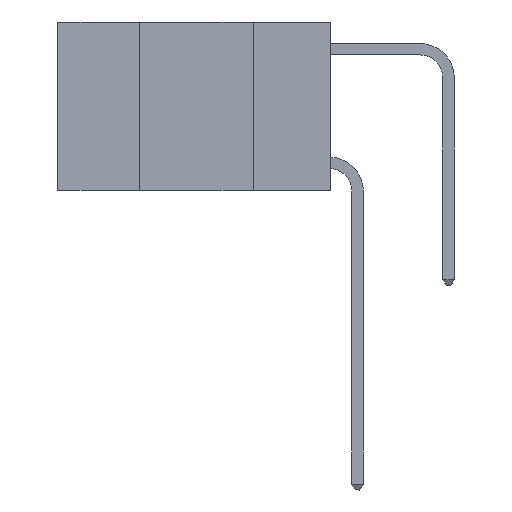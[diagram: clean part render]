
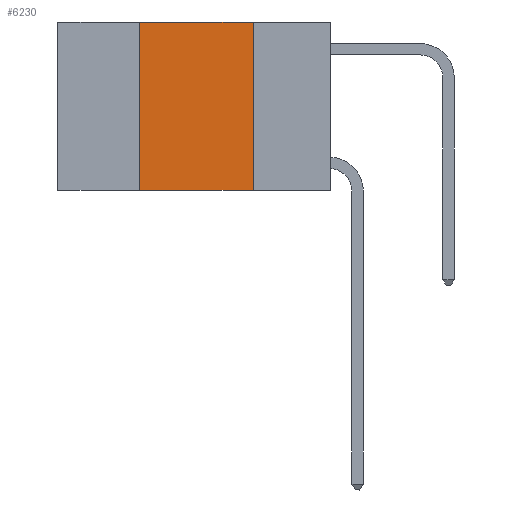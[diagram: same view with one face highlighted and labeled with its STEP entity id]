
A CAD part, left-side view. The second image highlights one B-rep face of the part: STEP entity #6230.
In plain terms, the highlighted planar face has unit normal (-1, 0, 0).
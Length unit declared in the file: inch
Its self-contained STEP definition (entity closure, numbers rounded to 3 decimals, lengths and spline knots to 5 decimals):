
#684 = CARTESIAN_POINT ( 'NONE',  ( 0., 0.6, 0. ) ) ;
#735 = CARTESIAN_POINT ( 'NONE',  ( 0., 0.42, -0.37 ) ) ;
#1099 = CARTESIAN_POINT ( 'NONE',  ( 0., 0.42, 0. ) ) ;
#1864 = EDGE_CURVE ( 'NONE', #15162, #2435, #2311, .T. ) ;
#2311 = LINE ( 'NONE', #20607, #16480 ) ;
#2326 = EDGE_CURVE ( 'NONE', #14271, #21335, #17048, .T. ) ;
#2435 = VERTEX_POINT ( 'NONE', #18611 ) ;
#2950 = VECTOR ( 'NONE', #8205, 39.37008 ) ;
#4415 = DIRECTION ( 'NONE',  ( 0., 0., -1. ) ) ;
#5647 = VECTOR ( 'NONE', #9096, 39.37008 ) ;
#5906 = EDGE_LOOP ( 'NONE', ( #21731, #22476, #23707, #12818 ) ) ;
#5960 = EDGE_CURVE ( 'NONE', #14271, #2435, #19722, .T. ) ;
#6230 = ADVANCED_FACE ( 'NONE', ( #9090 ), #20856, .F. ) ;
#6688 = VECTOR ( 'NONE', #23633, 39.37008 ) ;
#8205 = DIRECTION ( 'NONE',  ( 0., -1., 0. ) ) ;
#8472 = LINE ( 'NONE', #684, #2950 ) ;
#9090 = FACE_OUTER_BOUND ( 'NONE', #5906, .T. ) ;
#9096 = DIRECTION ( 'NONE',  ( 0., -1., 0. ) ) ;
#12818 = ORIENTED_EDGE ( 'NONE', *, *, #5960, .T. ) ;
#13279 = CARTESIAN_POINT ( 'NONE',  ( 0., 0.17, 0. ) ) ;
#14271 = VERTEX_POINT ( 'NONE', #735 ) ;
#15162 = VERTEX_POINT ( 'NONE', #13279 ) ;
#15457 = DIRECTION ( 'NONE',  ( 1., 0., 0. ) ) ;
#16480 = VECTOR ( 'NONE', #18806, 39.37008 ) ;
#17048 = LINE ( 'NONE', #21842, #6688 ) ;
#18611 = CARTESIAN_POINT ( 'NONE',  ( 0., 0.17, -0.37 ) ) ;
#18806 = DIRECTION ( 'NONE',  ( 0., 0., -1. ) ) ;
#19038 = CARTESIAN_POINT ( 'NONE',  ( 0., 0.6, 0. ) ) ;
#19722 = LINE ( 'NONE', #20061, #5647 ) ;
#20061 = CARTESIAN_POINT ( 'NONE',  ( 0., 0.6, -0.37 ) ) ;
#20607 = CARTESIAN_POINT ( 'NONE',  ( 0., 0.17, 0. ) ) ;
#20856 = PLANE ( 'NONE',  #21449 ) ;
#21199 = EDGE_CURVE ( 'NONE', #21335, #15162, #8472, .T. ) ;
#21335 = VERTEX_POINT ( 'NONE', #1099 ) ;
#21449 = AXIS2_PLACEMENT_3D ( 'NONE', #19038, #15457, #4415 ) ;
#21731 = ORIENTED_EDGE ( 'NONE', *, *, #1864, .F. ) ;
#21842 = CARTESIAN_POINT ( 'NONE',  ( 0., 0.42, 0. ) ) ;
#22476 = ORIENTED_EDGE ( 'NONE', *, *, #21199, .F. ) ;
#23633 = DIRECTION ( 'NONE',  ( 0., 0., 1. ) ) ;
#23707 = ORIENTED_EDGE ( 'NONE', *, *, #2326, .F. ) ;
